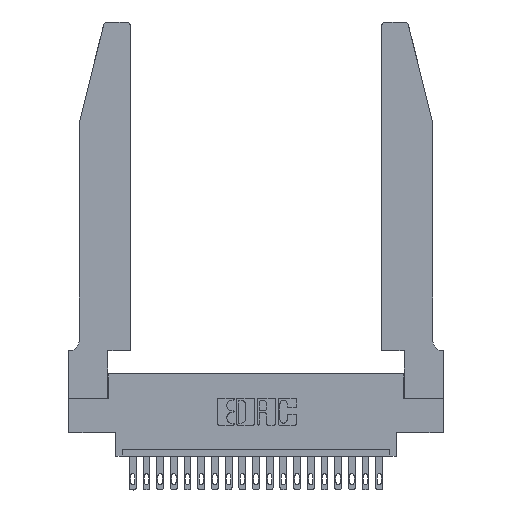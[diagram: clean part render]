
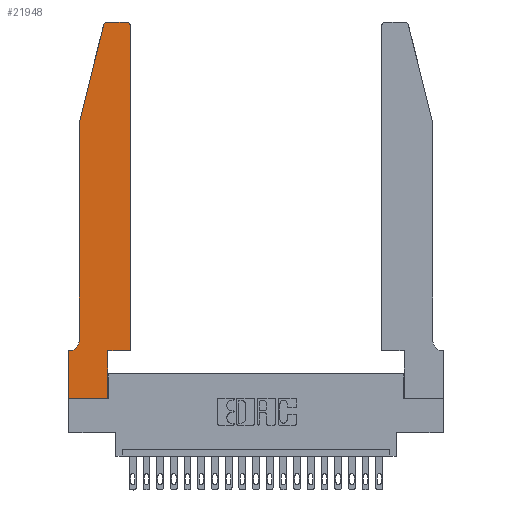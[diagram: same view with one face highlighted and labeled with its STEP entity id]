
A CAD part, top view. The second image highlights one B-rep face of the part: STEP entity #21948.
In plain terms, the highlighted planar face has unit normal (0, 0, 1).
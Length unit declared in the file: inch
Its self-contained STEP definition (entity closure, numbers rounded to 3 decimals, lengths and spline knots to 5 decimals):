
#604 = DIRECTION ( 'NONE',  ( -0.239, -0.971, 0. ) ) ;
#627 = CARTESIAN_POINT ( 'NONE',  ( 0.4505, 0.35, 0.37 ) ) ;
#980 = CARTESIAN_POINT ( 'NONE',  ( 0.2605, 2.75, 0.37 ) ) ;
#1017 = CIRCLE ( 'NONE', #6644, 0.03 ) ;
#1066 = ORIENTED_EDGE ( 'NONE', *, *, #5347, .T. ) ;
#1200 = CARTESIAN_POINT ( 'NONE',  ( 0., 0., 0.37 ) ) ;
#2103 = CARTESIAN_POINT ( 'NONE',  ( 0.284, 2.72, 0.37 ) ) ;
#2107 = VECTOR ( 'NONE', #604, 39.37008 ) ;
#2412 = CARTESIAN_POINT ( 'NONE',  ( 0.0755, 2., 0.37 ) ) ;
#2741 = DIRECTION ( 'NONE',  ( 0., 0., 1. ) ) ;
#2967 = VERTEX_POINT ( 'NONE', #13740 ) ;
#2986 = DIRECTION ( 'NONE',  ( 1., 0., 0. ) ) ;
#3134 = DIRECTION ( 'NONE',  ( 0., -1., 0. ) ) ;
#3305 = CARTESIAN_POINT ( 'NONE',  ( 0., 0., 0.37 ) ) ;
#3370 = VERTEX_POINT ( 'NONE', #13659 ) ;
#3549 = LINE ( 'NONE', #627, #10272 ) ;
#3794 = EDGE_CURVE ( 'NONE', #3370, #7629, #8061, .T. ) ;
#3991 = CARTESIAN_POINT ( 'NONE',  ( 0.2865, 0.35, 0.37 ) ) ;
#4113 = ORIENTED_EDGE ( 'NONE', *, *, #9687, .T. ) ;
#4412 = DIRECTION ( 'NONE',  ( -1., 0., 0. ) ) ;
#4453 = DIRECTION ( 'NONE',  ( 1., 0., 0. ) ) ;
#4454 = EDGE_CURVE ( 'NONE', #7629, #10566, #16892, .T. ) ;
#4588 = EDGE_CURVE ( 'NONE', #5327, #15938, #6435, .T. ) ;
#4811 = VECTOR ( 'NONE', #12715, 39.37008 ) ;
#5327 = VERTEX_POINT ( 'NONE', #15584 ) ;
#5347 = EDGE_CURVE ( 'NONE', #20553, #2967, #11197, .T. ) ;
#5576 = LINE ( 'NONE', #20255, #10668 ) ;
#5828 = LINE ( 'NONE', #980, #20590 ) ;
#6385 = CARTESIAN_POINT ( 'NONE',  ( 0.25487, 2.72718, 0.37 ) ) ;
#6435 = LINE ( 'NONE', #3991, #17435 ) ;
#6475 = VERTEX_POINT ( 'NONE', #16893 ) ;
#6604 = AXIS2_PLACEMENT_3D ( 'NONE', #7834, #2741, #4453 ) ;
#6618 = DIRECTION ( 'NONE',  ( 0., -1., 0. ) ) ;
#6644 = AXIS2_PLACEMENT_3D ( 'NONE', #2103, #10916, #10843 ) ;
#6816 = AXIS2_PLACEMENT_3D ( 'NONE', #7338, #10726, #19433 ) ;
#7140 = EDGE_CURVE ( 'NONE', #9578, #5327, #15414, .T. ) ;
#7338 = CARTESIAN_POINT ( 'NONE',  ( 0., 0.35, 0.37 ) ) ;
#7439 = CARTESIAN_POINT ( 'NONE',  ( 0.2865, 0.35, 0.37 ) ) ;
#7629 = VERTEX_POINT ( 'NONE', #9031 ) ;
#7658 = CARTESIAN_POINT ( 'NONE',  ( 0.0055, 0.42, 0.37 ) ) ;
#7793 = VECTOR ( 'NONE', #2986, 39.37008 ) ;
#7834 = CARTESIAN_POINT ( 'NONE',  ( 0.4205, 2.72, 0.37 ) ) ;
#7994 = ORIENTED_EDGE ( 'NONE', *, *, #3794, .T. ) ;
#8061 = CIRCLE ( 'NONE', #10868, 0.07 ) ;
#8234 = ORIENTED_EDGE ( 'NONE', *, *, #18868, .T. ) ;
#8705 = EDGE_CURVE ( 'NONE', #20729, #11335, #3549, .T. ) ;
#8796 = CARTESIAN_POINT ( 'NONE',  ( 0.4505, 0.35, 0.37 ) ) ;
#9030 = VECTOR ( 'NONE', #18378, 39.37008 ) ;
#9031 = CARTESIAN_POINT ( 'NONE',  ( 0.0055, 0.35, 0.37 ) ) ;
#9314 = CARTESIAN_POINT ( 'NONE',  ( 0.0755, 0.35, 0.37 ) ) ;
#9416 = DIRECTION ( 'NONE',  ( 0., 1., 0. ) ) ;
#9578 = VERTEX_POINT ( 'NONE', #16177 ) ;
#9687 = EDGE_CURVE ( 'NONE', #10566, #9578, #10744, .T. ) ;
#9741 = ORIENTED_EDGE ( 'NONE', *, *, #4588, .T. ) ;
#10040 = EDGE_LOOP ( 'NONE', ( #14192, #8234, #1066, #21579, #7994, #15918, #4113, #16687, #9741, #19542, #15557, #14078 ) ) ;
#10252 = EDGE_CURVE ( 'NONE', #15938, #20729, #17994, .T. ) ;
#10272 = VECTOR ( 'NONE', #9416, 39.37008 ) ;
#10566 = VERTEX_POINT ( 'NONE', #12314 ) ;
#10668 = VECTOR ( 'NONE', #3134, 39.37008 ) ;
#10726 = DIRECTION ( 'NONE',  ( 0., 0., 1. ) ) ;
#10744 = LINE ( 'NONE', #3305, #15545 ) ;
#10843 = DIRECTION ( 'NONE',  ( 1., 0., 0. ) ) ;
#10868 = AXIS2_PLACEMENT_3D ( 'NONE', #7658, #11096, #16516 ) ;
#10916 = DIRECTION ( 'NONE',  ( 0., 0., 1. ) ) ;
#11096 = DIRECTION ( 'NONE',  ( 0., 0., -1. ) ) ;
#11197 = LINE ( 'NONE', #2412, #2107 ) ;
#11335 = VERTEX_POINT ( 'NONE', #11382 ) ;
#11382 = CARTESIAN_POINT ( 'NONE',  ( 0.4505, 2.72, 0.37 ) ) ;
#12146 = EDGE_CURVE ( 'NONE', #2967, #3370, #5576, .T. ) ;
#12314 = CARTESIAN_POINT ( 'NONE',  ( 0., 0.35, 0.37 ) ) ;
#12353 = PLANE ( 'NONE',  #6816 ) ;
#12715 = DIRECTION ( 'NONE',  ( -1., 0., 0. ) ) ;
#13659 = CARTESIAN_POINT ( 'NONE',  ( 0.0755, 0.42, 0.37 ) ) ;
#13740 = CARTESIAN_POINT ( 'NONE',  ( 0.0755, 2., 0.37 ) ) ;
#13904 = CIRCLE ( 'NONE', #6604, 0.03 ) ;
#14078 = ORIENTED_EDGE ( 'NONE', *, *, #17692, .T. ) ;
#14192 = ORIENTED_EDGE ( 'NONE', *, *, #19020, .T. ) ;
#15068 = CARTESIAN_POINT ( 'NONE',  ( 0.4205, 2.75, 0.37 ) ) ;
#15414 = LINE ( 'NONE', #1200, #9030 ) ;
#15545 = VECTOR ( 'NONE', #6618, 39.37008 ) ;
#15557 = ORIENTED_EDGE ( 'NONE', *, *, #8705, .T. ) ;
#15584 = CARTESIAN_POINT ( 'NONE',  ( 0.2865, 0., 0.37 ) ) ;
#15918 = ORIENTED_EDGE ( 'NONE', *, *, #4454, .T. ) ;
#15938 = VERTEX_POINT ( 'NONE', #7439 ) ;
#16177 = CARTESIAN_POINT ( 'NONE',  ( 0., 0., 0.37 ) ) ;
#16451 = FACE_OUTER_BOUND ( 'NONE', #10040, .T. ) ;
#16516 = DIRECTION ( 'NONE',  ( -1., 0., 0. ) ) ;
#16687 = ORIENTED_EDGE ( 'NONE', *, *, #7140, .T. ) ;
#16892 = LINE ( 'NONE', #9314, #4811 ) ;
#16893 = CARTESIAN_POINT ( 'NONE',  ( 0.284, 2.75, 0.37 ) ) ;
#17435 = VECTOR ( 'NONE', #19242, 39.37008 ) ;
#17692 = EDGE_CURVE ( 'NONE', #11335, #20010, #13904, .T. ) ;
#17994 = LINE ( 'NONE', #21737, #7793 ) ;
#18378 = DIRECTION ( 'NONE',  ( 1., 0., 0. ) ) ;
#18868 = EDGE_CURVE ( 'NONE', #6475, #20553, #1017, .T. ) ;
#19020 = EDGE_CURVE ( 'NONE', #20010, #6475, #5828, .T. ) ;
#19242 = DIRECTION ( 'NONE',  ( 0., 1., 0. ) ) ;
#19433 = DIRECTION ( 'NONE',  ( 1., 0., 0. ) ) ;
#19542 = ORIENTED_EDGE ( 'NONE', *, *, #10252, .T. ) ;
#20010 = VERTEX_POINT ( 'NONE', #15068 ) ;
#20255 = CARTESIAN_POINT ( 'NONE',  ( 0.0755, 2., 0.37 ) ) ;
#20553 = VERTEX_POINT ( 'NONE', #6385 ) ;
#20590 = VECTOR ( 'NONE', #4412, 39.37008 ) ;
#20729 = VERTEX_POINT ( 'NONE', #8796 ) ;
#21579 = ORIENTED_EDGE ( 'NONE', *, *, #12146, .T. ) ;
#21737 = CARTESIAN_POINT ( 'NONE',  ( 0.4505, 0.35, 0.37 ) ) ;
#21948 = ADVANCED_FACE ( 'NONE', ( #16451 ), #12353, .T. ) ;
